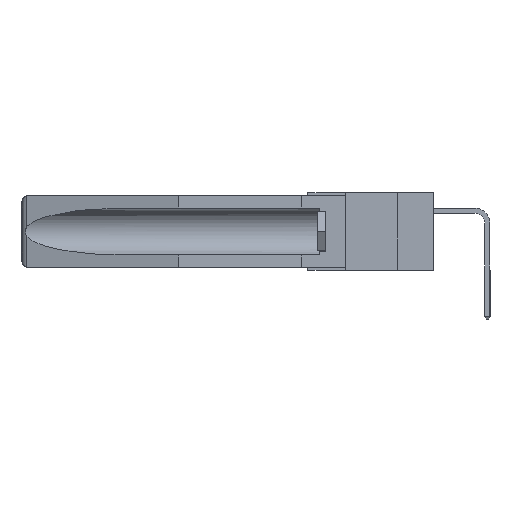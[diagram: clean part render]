
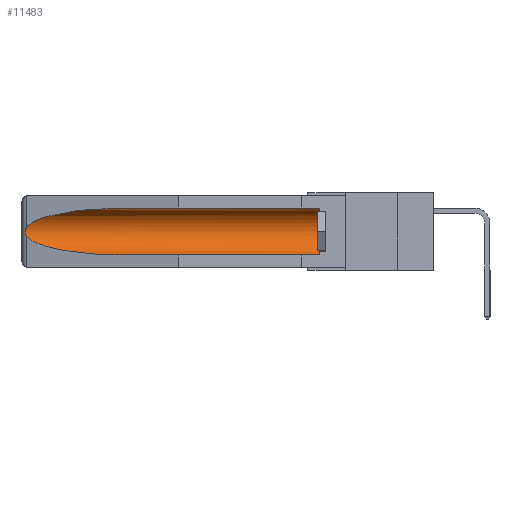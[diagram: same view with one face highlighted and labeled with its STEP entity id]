
A CAD part, left-side view. The second image highlights one B-rep face of the part: STEP entity #11483.
In plain terms, the highlighted cylindrical face has radius 2.857 mm (diameter 5.715 mm), a partial arc.
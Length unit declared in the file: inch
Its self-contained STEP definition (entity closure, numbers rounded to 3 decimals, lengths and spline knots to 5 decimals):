
#502 = LINE ( 'NONE', #2665, #3815 ) ;
#512 = VERTEX_POINT ( 'NONE', #15372 ) ;
#568 = DIRECTION ( 'NONE',  ( 0., -1., 0. ) ) ;
#805 = CARTESIAN_POINT ( 'NONE',  ( 0.2673, 1.53269, -0.17917 ) ) ;
#841 = EDGE_CURVE ( 'NONE', #2638, #8872, #6346, .T. ) ;
#919 =( BOUNDED_CURVE ( )  B_SPLINE_CURVE ( 3, ( #14054, #12736, #1813, #5307 ),
 .UNSPECIFIED., .F., .T. ) 
 B_SPLINE_CURVE_WITH_KNOTS ( ( 4, 4 ),
 ( 0.1948, 1.5708 ),
 .UNSPECIFIED. ) 
 CURVE ( )  GEOMETRIC_REPRESENTATION_ITEM ( )  RATIONAL_B_SPLINE_CURVE ( ( 1., 0.848, 0.848, 1. ) ) 
 REPRESENTATION_ITEM ( '' )  );
#1307 = AXIS2_PLACEMENT_3D ( 'NONE', #4014, #12671, #5233 ) ;
#1601 = VECTOR ( 'NONE', #1769, 39.37008 ) ;
#1632 = CARTESIAN_POINT ( 'NONE',  ( 0.26537, 1.52718, -0.14972 ) ) ;
#1769 = DIRECTION ( 'NONE',  ( 0., 1., 0. ) ) ;
#1813 = CARTESIAN_POINT ( 'NONE',  ( 0.21114, 1.30732, -0.284 ) ) ;
#2387 = ORIENTED_EDGE ( 'NONE', *, *, #11930, .F. ) ;
#2638 = VERTEX_POINT ( 'NONE', #7835 ) ;
#2665 = CARTESIAN_POINT ( 'NONE',  ( 0.155, -0.30754, -0.284 ) ) ;
#3019 = ORIENTED_EDGE ( 'NONE', *, *, #841, .T. ) ;
#3374 = AXIS2_PLACEMENT_3D ( 'NONE', #8776, #568, #4303 ) ;
#3423 = CIRCLE ( 'NONE', #3374, 0.1125 ) ;
#3815 = VECTOR ( 'NONE', #15004, 39.37008 ) ;
#3895 = EDGE_CURVE ( 'NONE', #4505, #2638, #7346, .T. ) ;
#3965 = EDGE_CURVE ( 'NONE', #8872, #4381, #8525, .T. ) ;
#4014 = CARTESIAN_POINT ( 'NONE',  ( 0.155, -0.30754, -0.1715 ) ) ;
#4303 = DIRECTION ( 'NONE',  ( 0., 0., 1. ) ) ;
#4381 = VERTEX_POINT ( 'NONE', #8619 ) ;
#4505 = VERTEX_POINT ( 'NONE', #5790 ) ;
#4535 = CARTESIAN_POINT ( 'NONE',  ( 0.26537, 1.52718, -0.19328 ) ) ;
#5233 = DIRECTION ( 'NONE',  ( 0., 0., 1. ) ) ;
#5307 = CARTESIAN_POINT ( 'NONE',  ( 0.155, 1.07973, -0.284 ) ) ;
#5723 = CARTESIAN_POINT ( 'NONE',  ( 0.26654, 1.53092, -0.15636 ) ) ;
#5768 = EDGE_CURVE ( 'NONE', #512, #4505, #3423, .T. ) ;
#5790 = CARTESIAN_POINT ( 'NONE',  ( 0.155, 0.126, -0.059 ) ) ;
#6346 =( BOUNDED_CURVE ( )  B_SPLINE_CURVE ( 3, ( #7675, #14046, #6410, #1632 ),
 .UNSPECIFIED., .F., .T. ) 
 B_SPLINE_CURVE_WITH_KNOTS ( ( 4, 4 ),
 ( 4.71239, 6.08839 ),
 .UNSPECIFIED. ) 
 CURVE ( )  GEOMETRIC_REPRESENTATION_ITEM ( )  RATIONAL_B_SPLINE_CURVE ( ( 1., 0.848, 0.848, 1. ) ) 
 REPRESENTATION_ITEM ( '' )  );
#6410 = CARTESIAN_POINT ( 'NONE',  ( 0.25451, 1.48313, -0.09465 ) ) ;
#6760 = CARTESIAN_POINT ( 'NONE',  ( 0.155, -0.30754, -0.059 ) ) ;
#6965 = CARTESIAN_POINT ( 'NONE',  ( 0.26655, 1.53094, -0.18657 ) ) ;
#7346 = LINE ( 'NONE', #6760, #1601 ) ;
#7675 = CARTESIAN_POINT ( 'NONE',  ( 0.155, 1.07973, -0.059 ) ) ;
#7682 = EDGE_CURVE ( 'NONE', #4381, #10968, #919, .T. ) ;
#7740 = CARTESIAN_POINT ( 'NONE',  ( 0.26537, 1.52718, -0.14972 ) ) ;
#7835 = CARTESIAN_POINT ( 'NONE',  ( 0.155, 1.07973, -0.059 ) ) ;
#8156 = CARTESIAN_POINT ( 'NONE',  ( 0.2675, 1.53308, -0.17534 ) ) ;
#8525 = B_SPLINE_CURVE_WITH_KNOTS ( 'NONE', 3,
 ( #9500, #15741, #5723, #13213, #14326, #8156, #805, #6965, #9395, #4535 ),
 .UNSPECIFIED., .F., .F.,
 ( 4, 2, 2, 2, 4 ),
 ( 0., 0.00029, 0.00058, 0.00087, 0.00117 ),
 .UNSPECIFIED. ) ;
#8619 = CARTESIAN_POINT ( 'NONE',  ( 0.26537, 1.52718, -0.19328 ) ) ;
#8776 = CARTESIAN_POINT ( 'NONE',  ( 0.155, 0.126, -0.1715 ) ) ;
#8872 = VERTEX_POINT ( 'NONE', #7740 ) ;
#9395 = CARTESIAN_POINT ( 'NONE',  ( 0.26597, 1.5296, -0.19026 ) ) ;
#9400 = CARTESIAN_POINT ( 'NONE',  ( 0.155, 1.07973, -0.284 ) ) ;
#9500 = CARTESIAN_POINT ( 'NONE',  ( 0.26537, 1.52718, -0.14972 ) ) ;
#9675 = CYLINDRICAL_SURFACE ( 'NONE', #1307, 0.1125 ) ;
#10968 = VERTEX_POINT ( 'NONE', #9400 ) ;
#11483 = ADVANCED_FACE ( 'NONE', ( #11643 ), #9675, .F. ) ;
#11643 = FACE_OUTER_BOUND ( 'NONE', #14910, .T. ) ;
#11930 = EDGE_CURVE ( 'NONE', #512, #10968, #502, .T. ) ;
#12671 = DIRECTION ( 'NONE',  ( 0., 1., 0. ) ) ;
#12736 = CARTESIAN_POINT ( 'NONE',  ( 0.25451, 1.48313, -0.24835 ) ) ;
#12868 = ORIENTED_EDGE ( 'NONE', *, *, #5768, .T. ) ;
#13213 = CARTESIAN_POINT ( 'NONE',  ( 0.2673, 1.5327, -0.16383 ) ) ;
#13503 = ORIENTED_EDGE ( 'NONE', *, *, #3965, .T. ) ;
#13802 = ORIENTED_EDGE ( 'NONE', *, *, #3895, .T. ) ;
#14046 = CARTESIAN_POINT ( 'NONE',  ( 0.21114, 1.30732, -0.059 ) ) ;
#14054 = CARTESIAN_POINT ( 'NONE',  ( 0.26537, 1.52718, -0.19328 ) ) ;
#14326 = CARTESIAN_POINT ( 'NONE',  ( 0.2675, 1.53308, -0.16763 ) ) ;
#14910 = EDGE_LOOP ( 'NONE', ( #3019, #13503, #15039, #2387, #12868, #13802 ) ) ;
#15004 = DIRECTION ( 'NONE',  ( 0., 1., 0. ) ) ;
#15039 = ORIENTED_EDGE ( 'NONE', *, *, #7682, .T. ) ;
#15372 = CARTESIAN_POINT ( 'NONE',  ( 0.155, 0.126, -0.284 ) ) ;
#15741 = CARTESIAN_POINT ( 'NONE',  ( 0.26597, 1.52961, -0.15275 ) ) ;
